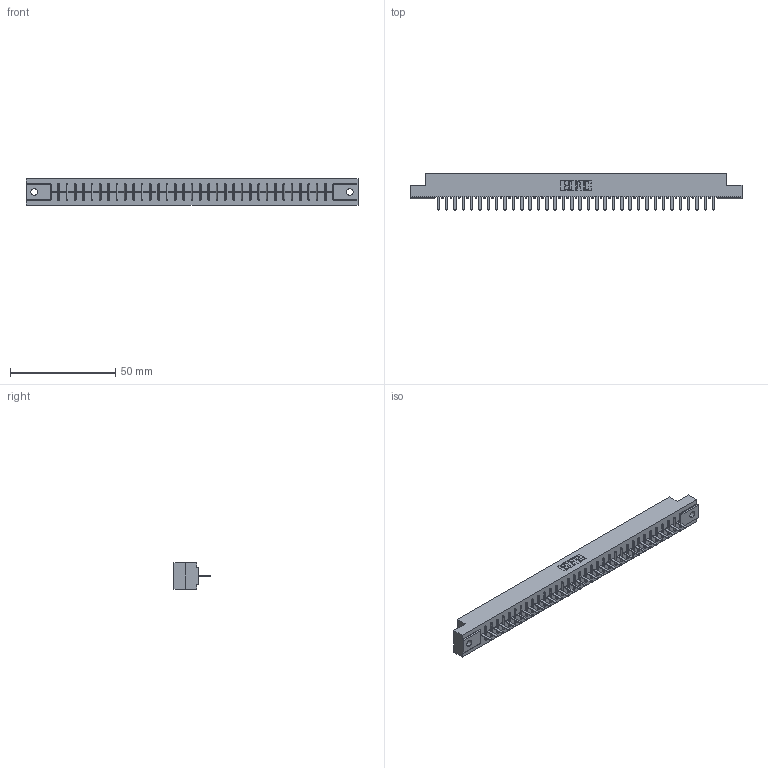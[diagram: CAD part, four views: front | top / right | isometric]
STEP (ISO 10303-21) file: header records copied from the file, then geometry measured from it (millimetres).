
FILE_DESCRIPTION (( 'STEP AP203' ), '1' );
FILE_NAME ('316-034-520-102.STEP', '2018-07-31T04:03:20', ( '' ), ( '' ), 'SwSTEP 2.0', 'SolidWorks 2016', '' );
FILE_SCHEMA (( 'CONFIG_CONTROL_DESIGN' ));
Length unit declared in the file: inch
Products named in the file (3): 306 Part_.128 Dia; 306-290-001_120; 316-034-520-102
Assembly tree (35 placements, depth 2):
  316-034-520-102
    306 Part_.128 Dia
    306-290-001_120  x34
Bounding box: 157.73 x 17.12 x 12.7 mm (x, y, z)
Volume: 17345 mm3; surface area: 17443.1 mm2
Topology: 35 solids, 35 shells, 2496 faces, 7014 edges, 4492 vertices
Faces by surface type: plane 1666, cylinder 694, sphere 136
Entity records: 32701 total; most frequent: CARTESIAN_POINT 5489, ORIENTED_EDGE 5440, DIRECTION 5414, EDGE_CURVE 2720, LINE 2124, VECTOR 2124, VERTEX_POINT 1720, AXIS2_PLACEMENT_3D 1645
